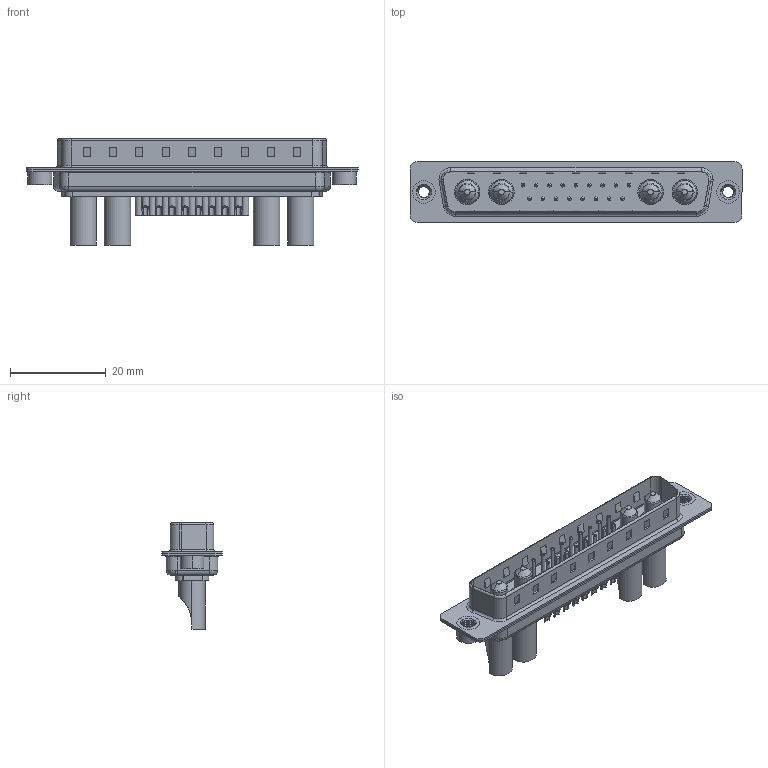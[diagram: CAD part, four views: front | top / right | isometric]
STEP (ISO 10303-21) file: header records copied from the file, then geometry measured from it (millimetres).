
FILE_DESCRIPTION (( 'STEP AP203' ), '1' );
FILE_NAME ('627-21W4222-4TA.STEP', '2019-06-26T12:12:42', ( '' ), ( '' ), 'SwSTEP 2.0', 'SolidWorks 2016', '' );
FILE_SCHEMA (( 'CONFIG_CONTROL_DESIGN' ));
Length unit declared in the file: millimetre
Products named in the file (8): 627Combo Shell Front_37 Contacts; 627Combo Housing_21W4; 627Combo Shell Rear_37 Contacts; 627Combo Contact Row 1_22; 627Combo Threaded Rivet_A; Power Pin_40A SC; 627-21W4222-4TA; 627Combo Contact Row 2_22
Assembly tree (26 placements, depth 2):
  627-21W4222-4TA
    627Combo Housing_21W4
    627Combo Shell Rear_37 Contacts
    627Combo Shell Front_37 Contacts
    627Combo Threaded Rivet_A  x2
    Power Pin_40A SC  x4
    627Combo Contact Row 1_22  x9
    627Combo Contact Row 2_22  x8
Bounding box: 69.3 x 12.6 x 22.3 mm (x, y, z)
Volume: 4229.9 mm3; surface area: 9835 mm2
Topology: 30 solids, 30 shells, 1211 faces, 2863 edges, 1757 vertices
Faces by surface type: cylinder 495, plane 404, torus 228, cone 70, bspline 14
Entity records: 22020 total; most frequent: CARTESIAN_POINT 5231, DIRECTION 3405, ORIENTED_EDGE 3070, EDGE_CURVE 1535, AXIS2_PLACEMENT_3D 1291, VERTEX_POINT 975, LINE 823, VECTOR 823
